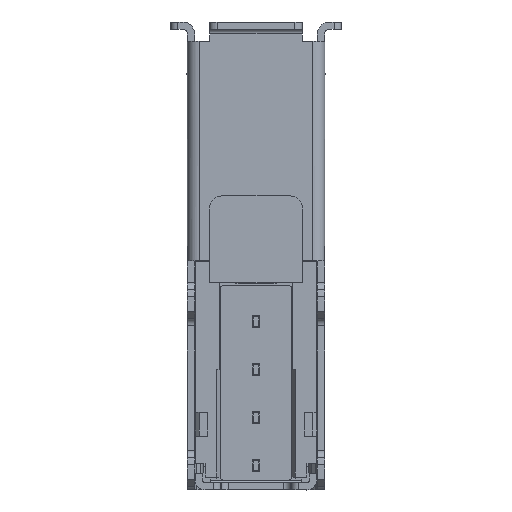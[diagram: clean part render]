
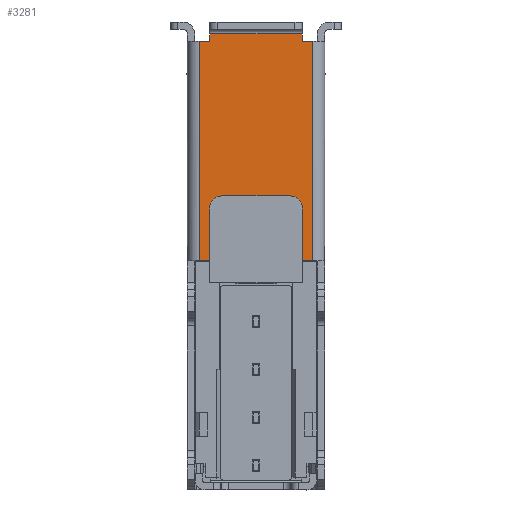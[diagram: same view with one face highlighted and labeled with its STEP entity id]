
A CAD part, front view. The second image highlights one B-rep face of the part: STEP entity #3281.
In plain terms, the highlighted planar face has unit normal (0, -1, 0).
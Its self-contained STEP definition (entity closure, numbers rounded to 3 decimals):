
#5 = VECTOR ( 'NONE', #28369, 1000. ) ;
#281 = CARTESIAN_POINT ( 'NONE',  ( 1.52, -6.55, 1. ) ) ;
#508 = ORIENTED_EDGE ( 'NONE', *, *, #3626, .F. ) ;
#682 = DIRECTION ( 'NONE',  ( -1., 0., 0. ) ) ;
#1085 = LINE ( 'NONE', #37850, #29483 ) ;
#1102 = DIRECTION ( 'NONE',  ( 1., 0., 0. ) ) ;
#1822 = CARTESIAN_POINT ( 'NONE',  ( 0.82, -6.55, -1. ) ) ;
#2279 = CARTESIAN_POINT ( 'NONE',  ( 1.52, -6.55, 0.75 ) ) ;
#2618 = LINE ( 'NONE', #17919, #34607 ) ;
#2918 = CARTESIAN_POINT ( 'NONE',  ( -3.305, -6.55, -1. ) ) ;
#2984 = LINE ( 'NONE', #27705, #34344 ) ;
#3281 = ADVANCED_FACE ( 'NONE', ( #15695 ), #19111, .F. ) ;
#3626 = EDGE_CURVE ( 'NONE', #21875, #33609, #11444, .T. ) ;
#4637 = ORIENTED_EDGE ( 'NONE', *, *, #9978, .F. ) ;
#4808 = EDGE_CURVE ( 'NONE', #5568, #9816, #10487, .T. ) ;
#5302 = VECTOR ( 'NONE', #34936, 1000. ) ;
#5394 = DIRECTION ( 'NONE',  ( 0., 0., -1. ) ) ;
#5568 = VERTEX_POINT ( 'NONE', #28066 ) ;
#5937 = CARTESIAN_POINT ( 'NONE',  ( 1.77, -6.55, 0.75 ) ) ;
#7111 = DIRECTION ( 'NONE',  ( 0., 0., -1. ) ) ;
#7637 = DIRECTION ( 'NONE',  ( 1., 0., 0. ) ) ;
#7680 = ORIENTED_EDGE ( 'NONE', *, *, #13962, .F. ) ;
#7720 = VERTEX_POINT ( 'NONE', #22536 ) ;
#7833 = LINE ( 'NONE', #29335, #21508 ) ;
#9271 = CARTESIAN_POINT ( 'NONE',  ( 1.77, -6.55, -0.75 ) ) ;
#9633 = DIRECTION ( 'NONE',  ( 0., 0., 1. ) ) ;
#9816 = VERTEX_POINT ( 'NONE', #281 ) ;
#9978 = EDGE_CURVE ( 'NONE', #33609, #30890, #17232, .T. ) ;
#10190 = EDGE_CURVE ( 'NONE', #10608, #38010, #13476, .T. ) ;
#10487 = LINE ( 'NONE', #13903, #20421 ) ;
#10608 = VERTEX_POINT ( 'NONE', #25476 ) ;
#11070 = EDGE_CURVE ( 'NONE', #38010, #29747, #1085, .T. ) ;
#11444 = LINE ( 'NONE', #39342, #20995 ) ;
#11597 = AXIS2_PLACEMENT_3D ( 'NONE', #2279, #13961, #29416 ) ;
#13121 = LINE ( 'NONE', #32180, #5 ) ;
#13463 = CARTESIAN_POINT ( 'NONE',  ( -8.33, -6.55, 0.88 ) ) ;
#13476 = LINE ( 'NONE', #19110, #37090 ) ;
#13705 = DIRECTION ( 'NONE',  ( 1., 0., 0. ) ) ;
#13903 = CARTESIAN_POINT ( 'NONE',  ( -3.305, -6.55, 1. ) ) ;
#13961 = DIRECTION ( 'NONE',  ( 0., 1., 0. ) ) ;
#13962 = EDGE_CURVE ( 'NONE', #24691, #32981, #13121, .T. ) ;
#13968 = DIRECTION ( 'NONE',  ( 0., 0., 1. ) ) ;
#14112 = ORIENTED_EDGE ( 'NONE', *, *, #29700, .F. ) ;
#14336 = CARTESIAN_POINT ( 'NONE',  ( 1.52, -6.55, -1. ) ) ;
#14761 = VECTOR ( 'NONE', #682, 1000. ) ;
#15026 = ORIENTED_EDGE ( 'NONE', *, *, #11070, .F. ) ;
#15515 = VECTOR ( 'NONE', #15759, 1000. ) ;
#15695 = FACE_OUTER_BOUND ( 'NONE', #30728, .T. ) ;
#15759 = DIRECTION ( 'NONE',  ( 0., 0., 1. ) ) ;
#15792 = LINE ( 'NONE', #2918, #14761 ) ;
#16043 = CARTESIAN_POINT ( 'NONE',  ( 0.82, -6.55, -2.36 ) ) ;
#16150 = CARTESIAN_POINT ( 'NONE',  ( -8.33, -6.55, -0.88 ) ) ;
#16205 = LINE ( 'NONE', #28656, #17044 ) ;
#16241 = ORIENTED_EDGE ( 'NONE', *, *, #22669, .F. ) ;
#16645 = ORIENTED_EDGE ( 'NONE', *, *, #29976, .F. ) ;
#16903 = ORIENTED_EDGE ( 'NONE', *, *, #4808, .F. ) ;
#17044 = VECTOR ( 'NONE', #1102, 1000. ) ;
#17127 = AXIS2_PLACEMENT_3D ( 'NONE', #27733, #31532, #9633 ) ;
#17142 = EDGE_CURVE ( 'NONE', #24691, #24102, #2618, .T. ) ;
#17232 = CIRCLE ( 'NONE', #30686, 0.25 ) ;
#17919 = CARTESIAN_POINT ( 'NONE',  ( 0.82, -6.55, 0. ) ) ;
#18767 = LINE ( 'NONE', #16150, #15515 ) ;
#19110 = CARTESIAN_POINT ( 'NONE',  ( -3.305, -6.55, -1.925 ) ) ;
#19111 = PLANE ( 'NONE',  #17127 ) ;
#19890 = LINE ( 'NONE', #13463, #5302 ) ;
#20116 = CARTESIAN_POINT ( 'NONE',  ( -8.63, -6.55, 1.925 ) ) ;
#20421 = VECTOR ( 'NONE', #13705, 1000. ) ;
#20499 = ORIENTED_EDGE ( 'NONE', *, *, #25965, .F. ) ;
#20501 = ORIENTED_EDGE ( 'NONE', *, *, #17142, .T. ) ;
#20612 = CIRCLE ( 'NONE', #11597, 0.25 ) ;
#20995 = VECTOR ( 'NONE', #5394, 1000. ) ;
#21508 = VECTOR ( 'NONE', #7637, 1000. ) ;
#21875 = VERTEX_POINT ( 'NONE', #5937 ) ;
#21938 = EDGE_CURVE ( 'NONE', #30890, #24102, #15792, .T. ) ;
#22536 = CARTESIAN_POINT ( 'NONE',  ( -8.33, -6.55, 2.36 ) ) ;
#22669 = EDGE_CURVE ( 'NONE', #9816, #21875, #20612, .T. ) ;
#22831 = ORIENTED_EDGE ( 'NONE', *, *, #10190, .F. ) ;
#24102 = VERTEX_POINT ( 'NONE', #1822 ) ;
#24197 = ORIENTED_EDGE ( 'NONE', *, *, #21938, .F. ) ;
#24691 = VERTEX_POINT ( 'NONE', #16043 ) ;
#25452 = ORIENTED_EDGE ( 'NONE', *, *, #35236, .F. ) ;
#25476 = CARTESIAN_POINT ( 'NONE',  ( -8.33, -6.55, -1.925 ) ) ;
#25965 = EDGE_CURVE ( 'NONE', #32981, #10608, #18767, .T. ) ;
#26249 = VERTEX_POINT ( 'NONE', #39606 ) ;
#26958 = CARTESIAN_POINT ( 'NONE',  ( 1.52, -6.55, -0.75 ) ) ;
#27705 = CARTESIAN_POINT ( 'NONE',  ( 0.82, -6.55, 0.88 ) ) ;
#27733 = CARTESIAN_POINT ( 'NONE',  ( -3.305, -6.55, -0.88 ) ) ;
#28066 = CARTESIAN_POINT ( 'NONE',  ( 0.82, -6.55, 1. ) ) ;
#28369 = DIRECTION ( 'NONE',  ( -1., 0., 0. ) ) ;
#28531 = DIRECTION ( 'NONE',  ( -1., 0., 0. ) ) ;
#28656 = CARTESIAN_POINT ( 'NONE',  ( -3.305, -6.55, 1.925 ) ) ;
#28714 = ORIENTED_EDGE ( 'NONE', *, *, #30331, .F. ) ;
#29335 = CARTESIAN_POINT ( 'NONE',  ( -8.518, -6.55, 2.36 ) ) ;
#29416 = DIRECTION ( 'NONE',  ( 0., 0., -1. ) ) ;
#29483 = VECTOR ( 'NONE', #13968, 1000. ) ;
#29700 = EDGE_CURVE ( 'NONE', #7720, #26249, #7833, .T. ) ;
#29747 = VERTEX_POINT ( 'NONE', #20116 ) ;
#29976 = EDGE_CURVE ( 'NONE', #26249, #5568, #2984, .T. ) ;
#30076 = CARTESIAN_POINT ( 'NONE',  ( -8.63, -6.55, -1.925 ) ) ;
#30161 = DIRECTION ( 'NONE',  ( 0., 0., 1. ) ) ;
#30331 = EDGE_CURVE ( 'NONE', #29747, #39108, #16205, .T. ) ;
#30671 = CARTESIAN_POINT ( 'NONE',  ( -8.33, -6.55, 1.925 ) ) ;
#30686 = AXIS2_PLACEMENT_3D ( 'NONE', #26958, #32771, #7111 ) ;
#30728 = EDGE_LOOP ( 'NONE', ( #24197, #4637, #508, #16241, #16903, #16645, #14112, #25452, #28714, #15026, #22831, #20499, #7680, #20501 ) ) ;
#30890 = VERTEX_POINT ( 'NONE', #14336 ) ;
#31532 = DIRECTION ( 'NONE',  ( 0., 1., 0. ) ) ;
#31911 = CARTESIAN_POINT ( 'NONE',  ( -8.33, -6.55, -2.36 ) ) ;
#32180 = CARTESIAN_POINT ( 'NONE',  ( -8.518, -6.55, -2.36 ) ) ;
#32771 = DIRECTION ( 'NONE',  ( 0., 1., 0. ) ) ;
#32981 = VERTEX_POINT ( 'NONE', #31911 ) ;
#33609 = VERTEX_POINT ( 'NONE', #9271 ) ;
#33729 = DIRECTION ( 'NONE',  ( 0., 0., -1. ) ) ;
#34344 = VECTOR ( 'NONE', #33729, 1000. ) ;
#34607 = VECTOR ( 'NONE', #30161, 1000. ) ;
#34936 = DIRECTION ( 'NONE',  ( 0., 0., 1. ) ) ;
#35236 = EDGE_CURVE ( 'NONE', #39108, #7720, #19890, .T. ) ;
#37090 = VECTOR ( 'NONE', #28531, 1000. ) ;
#37850 = CARTESIAN_POINT ( 'NONE',  ( -8.63, -6.55, -0.88 ) ) ;
#38010 = VERTEX_POINT ( 'NONE', #30076 ) ;
#39108 = VERTEX_POINT ( 'NONE', #30671 ) ;
#39342 = CARTESIAN_POINT ( 'NONE',  ( 1.77, -6.55, -0.88 ) ) ;
#39606 = CARTESIAN_POINT ( 'NONE',  ( 0.82, -6.55, 2.36 ) ) ;
